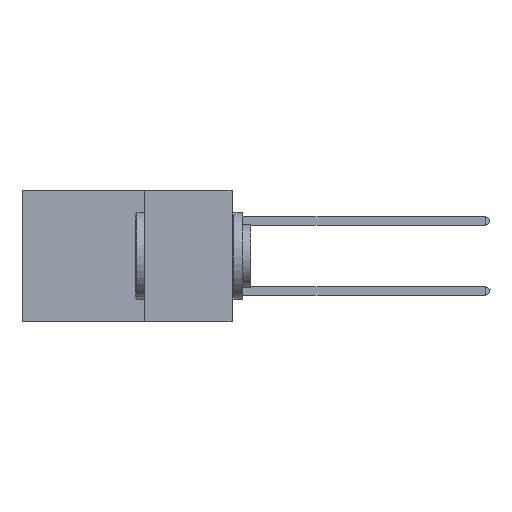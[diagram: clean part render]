
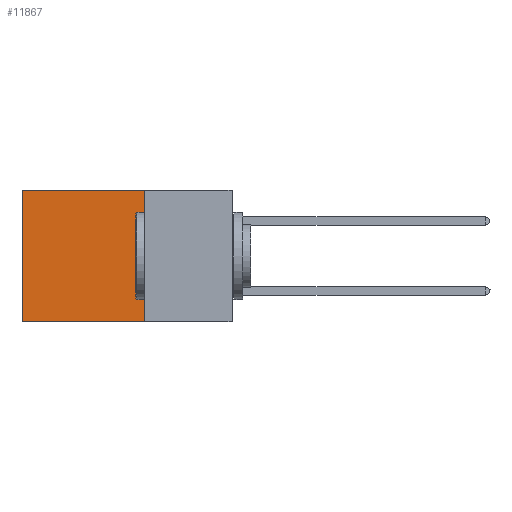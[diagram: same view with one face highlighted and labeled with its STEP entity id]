
A CAD part, left-side view. The second image highlights one B-rep face of the part: STEP entity #11867.
In plain terms, the highlighted planar face has unit normal (-1, 0, 0).
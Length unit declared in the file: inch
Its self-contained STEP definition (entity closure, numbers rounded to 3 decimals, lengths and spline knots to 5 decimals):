
#258 = PLANE ( 'NONE',  #9560 ) ;
#929 = CARTESIAN_POINT ( 'NONE',  ( 0.2875, 0.25, 0. ) ) ;
#1603 = EDGE_CURVE ( 'NONE', #16164, #13540, #4430, .T. ) ;
#1976 = CARTESIAN_POINT ( 'NONE',  ( 0.2875, 0.25, -0.375 ) ) ;
#2076 = DIRECTION ( 'NONE',  ( 0., 0., -1. ) ) ;
#2340 = EDGE_LOOP ( 'NONE', ( #11611, #11598, #5359, #13560 ) ) ;
#2410 = VECTOR ( 'NONE', #13970, 39.37008 ) ;
#2790 = DIRECTION ( 'NONE',  ( 0., 0., -1. ) ) ;
#4109 = DIRECTION ( 'NONE',  ( 1., 0., 0. ) ) ;
#4430 = LINE ( 'NONE', #8907, #14148 ) ;
#5359 = ORIENTED_EDGE ( 'NONE', *, *, #13610, .F. ) ;
#6022 = LINE ( 'NONE', #6387, #15377 ) ;
#6387 = CARTESIAN_POINT ( 'NONE',  ( 0.2875, 0.25, 0. ) ) ;
#7463 = FACE_OUTER_BOUND ( 'NONE', #2340, .T. ) ;
#7770 = CARTESIAN_POINT ( 'NONE',  ( 0.2875, 0.6, -0.375 ) ) ;
#7900 = CARTESIAN_POINT ( 'NONE',  ( 0.2875, 0.25, -0.375 ) ) ;
#7948 = VECTOR ( 'NONE', #2076, 39.37008 ) ;
#7989 = EDGE_CURVE ( 'NONE', #13165, #10042, #6022, .T. ) ;
#8907 = CARTESIAN_POINT ( 'NONE',  ( 0.2875, 0.25, -0.375 ) ) ;
#9560 = AXIS2_PLACEMENT_3D ( 'NONE', #7900, #4109, #2790 ) ;
#10042 = VERTEX_POINT ( 'NONE', #14827 ) ;
#10476 = CARTESIAN_POINT ( 'NONE',  ( 0.2875, 0.6, -0.375 ) ) ;
#10526 = EDGE_CURVE ( 'NONE', #10042, #13540, #11322, .T. ) ;
#11322 = LINE ( 'NONE', #7770, #2410 ) ;
#11513 = DIRECTION ( 'NONE',  ( 0., 1., 0. ) ) ;
#11598 = ORIENTED_EDGE ( 'NONE', *, *, #1603, .F. ) ;
#11611 = ORIENTED_EDGE ( 'NONE', *, *, #10526, .T. ) ;
#11867 = ADVANCED_FACE ( 'NONE', ( #7463 ), #258, .F. ) ;
#12733 = DIRECTION ( 'NONE',  ( 0., 1., 0. ) ) ;
#13165 = VERTEX_POINT ( 'NONE', #929 ) ;
#13540 = VERTEX_POINT ( 'NONE', #10476 ) ;
#13560 = ORIENTED_EDGE ( 'NONE', *, *, #7989, .T. ) ;
#13610 = EDGE_CURVE ( 'NONE', #13165, #16164, #15320, .T. ) ;
#13970 = DIRECTION ( 'NONE',  ( 0., 0., -1. ) ) ;
#14148 = VECTOR ( 'NONE', #12733, 39.37008 ) ;
#14827 = CARTESIAN_POINT ( 'NONE',  ( 0.2875, 0.6, 0. ) ) ;
#15320 = LINE ( 'NONE', #1976, #7948 ) ;
#15377 = VECTOR ( 'NONE', #11513, 39.37008 ) ;
#15889 = CARTESIAN_POINT ( 'NONE',  ( 0.2875, 0.25, -0.375 ) ) ;
#16164 = VERTEX_POINT ( 'NONE', #15889 ) ;
